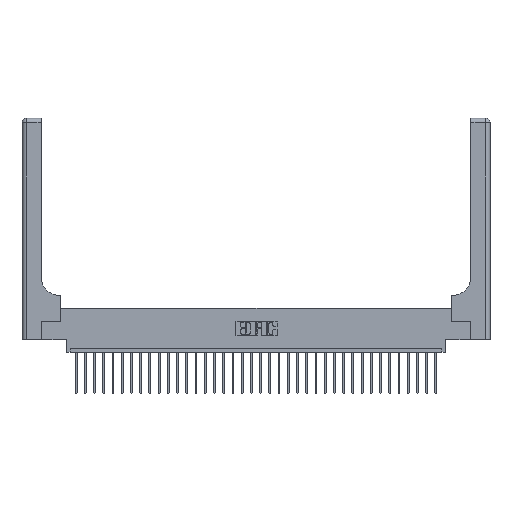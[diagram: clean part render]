
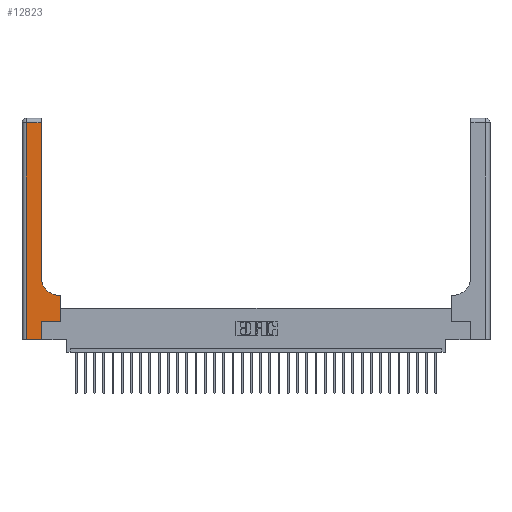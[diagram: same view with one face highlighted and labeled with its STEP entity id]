
A CAD part, top view. The second image highlights one B-rep face of the part: STEP entity #12823.
In plain terms, the highlighted planar face has unit normal (0, 0, 1).
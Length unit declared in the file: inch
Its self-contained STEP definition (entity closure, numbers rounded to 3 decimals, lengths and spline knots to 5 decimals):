
#86 = LINE ( 'NONE', #18781, #7908 ) ;
#174 = DIRECTION ( 'NONE',  ( -1., 0., 0. ) ) ;
#905 = PLANE ( 'NONE',  #30037 ) ;
#2286 = LINE ( 'NONE', #4970, #17020 ) ;
#3731 = DIRECTION ( 'NONE',  ( -1., 0., 0. ) ) ;
#4066 = CARTESIAN_POINT ( 'NONE',  ( 0.26, 2.94, 0.37 ) ) ;
#4112 = VERTEX_POINT ( 'NONE', #7474 ) ;
#4348 = LINE ( 'NONE', #20897, #28517 ) ;
#4426 = VERTEX_POINT ( 'NONE', #4066 ) ;
#4915 = CARTESIAN_POINT ( 'NONE',  ( 0.06, 2.94, 0.37 ) ) ;
#4970 = CARTESIAN_POINT ( 'NONE',  ( 0.528, 0.25, 0.37 ) ) ;
#6006 = DIRECTION ( 'NONE',  ( 0., 0., -1. ) ) ;
#6823 = VERTEX_POINT ( 'NONE', #7811 ) ;
#6849 = ORIENTED_EDGE ( 'NONE', *, *, #12622, .T. ) ;
#7474 = CARTESIAN_POINT ( 'NONE',  ( 0.265, 0., 0.37 ) ) ;
#7811 = CARTESIAN_POINT ( 'NONE',  ( 0.528, 0.25, 0.37 ) ) ;
#7908 = VECTOR ( 'NONE', #9663, 39.37008 ) ;
#8454 = EDGE_CURVE ( 'NONE', #21024, #4426, #19299, .T. ) ;
#9227 = CARTESIAN_POINT ( 'NONE',  ( 0.265, 0.25, 0.37 ) ) ;
#9582 = ORIENTED_EDGE ( 'NONE', *, *, #11792, .T. ) ;
#9663 = DIRECTION ( 'NONE',  ( 0., -1., 0. ) ) ;
#11144 = ORIENTED_EDGE ( 'NONE', *, *, #14262, .T. ) ;
#11792 = EDGE_CURVE ( 'NONE', #28270, #6823, #13527, .T. ) ;
#12622 = EDGE_CURVE ( 'NONE', #4112, #28270, #4348, .T. ) ;
#12823 = ADVANCED_FACE ( 'NONE', ( #29595 ), #905, .F. ) ;
#12825 = VERTEX_POINT ( 'NONE', #13071 ) ;
#12966 = VERTEX_POINT ( 'NONE', #19039 ) ;
#13030 = VECTOR ( 'NONE', #13961, 39.37008 ) ;
#13071 = CARTESIAN_POINT ( 'NONE',  ( 0.528, 0.6, 0.37 ) ) ;
#13268 = CIRCLE ( 'NONE', #25386, 0.25 ) ;
#13359 = VECTOR ( 'NONE', #27005, 39.37008 ) ;
#13527 = LINE ( 'NONE', #27594, #27817 ) ;
#13961 = DIRECTION ( 'NONE',  ( 0., 1., 0. ) ) ;
#14262 = EDGE_CURVE ( 'NONE', #4426, #24753, #20369, .T. ) ;
#14575 = EDGE_CURVE ( 'NONE', #6823, #12825, #2286, .T. ) ;
#15204 = ORIENTED_EDGE ( 'NONE', *, *, #19907, .T. ) ;
#15368 = CARTESIAN_POINT ( 'NONE',  ( 0., 2.94, 0.37 ) ) ;
#15503 = EDGE_CURVE ( 'NONE', #12966, #21024, #13268, .T. ) ;
#16274 = EDGE_CURVE ( 'NONE', #12825, #12966, #25276, .T. ) ;
#16343 = ORIENTED_EDGE ( 'NONE', *, *, #16274, .T. ) ;
#16352 = CARTESIAN_POINT ( 'NONE',  ( 0., 0., 0.37 ) ) ;
#16463 = ORIENTED_EDGE ( 'NONE', *, *, #14575, .T. ) ;
#17020 = VECTOR ( 'NONE', #26473, 39.37008 ) ;
#18781 = CARTESIAN_POINT ( 'NONE',  ( 0.06, 3., 0.37 ) ) ;
#19039 = CARTESIAN_POINT ( 'NONE',  ( 0.51, 0.6, 0.37 ) ) ;
#19051 = ORIENTED_EDGE ( 'NONE', *, *, #8454, .T. ) ;
#19299 = LINE ( 'NONE', #20740, #13030 ) ;
#19511 = EDGE_CURVE ( 'NONE', #24753, #30418, #86, .T. ) ;
#19907 = EDGE_CURVE ( 'NONE', #30418, #4112, #30331, .T. ) ;
#20080 = CARTESIAN_POINT ( 'NONE',  ( 0., 3., 0.37 ) ) ;
#20369 = LINE ( 'NONE', #15368, #13359 ) ;
#20678 = DIRECTION ( 'NONE',  ( 1., 0., 0. ) ) ;
#20740 = CARTESIAN_POINT ( 'NONE',  ( 0.26, 3., 0.37 ) ) ;
#20897 = CARTESIAN_POINT ( 'NONE',  ( 0.265, 0., 0.37 ) ) ;
#21024 = VERTEX_POINT ( 'NONE', #25613 ) ;
#21196 = CARTESIAN_POINT ( 'NONE',  ( 0.51, 0.85, 0.37 ) ) ;
#21583 = VECTOR ( 'NONE', #20678, 39.37008 ) ;
#22731 = VECTOR ( 'NONE', #174, 39.37008 ) ;
#22961 = EDGE_LOOP ( 'NONE', ( #19051, #11144, #27529, #15204, #6849, #9582, #16463, #16343, #30159 ) ) ;
#23328 = DIRECTION ( 'NONE',  ( 0., 1., 0. ) ) ;
#23730 = DIRECTION ( 'NONE',  ( 1., 0., 0. ) ) ;
#23828 = CARTESIAN_POINT ( 'NONE',  ( 0.26, 0.6, 0.37 ) ) ;
#24753 = VERTEX_POINT ( 'NONE', #4915 ) ;
#25276 = LINE ( 'NONE', #23828, #22731 ) ;
#25386 = AXIS2_PLACEMENT_3D ( 'NONE', #21196, #28212, #23730 ) ;
#25529 = DIRECTION ( 'NONE',  ( 1., 0., 0. ) ) ;
#25613 = CARTESIAN_POINT ( 'NONE',  ( 0.26, 0.85, 0.37 ) ) ;
#26473 = DIRECTION ( 'NONE',  ( 0., 1., 0. ) ) ;
#27005 = DIRECTION ( 'NONE',  ( -1., 0., 0. ) ) ;
#27529 = ORIENTED_EDGE ( 'NONE', *, *, #19511, .T. ) ;
#27594 = CARTESIAN_POINT ( 'NONE',  ( 0.265, 0.25, 0.37 ) ) ;
#27678 = CARTESIAN_POINT ( 'NONE',  ( 0.06, 0., 0.37 ) ) ;
#27817 = VECTOR ( 'NONE', #25529, 39.37008 ) ;
#28212 = DIRECTION ( 'NONE',  ( 0., 0., -1. ) ) ;
#28270 = VERTEX_POINT ( 'NONE', #9227 ) ;
#28517 = VECTOR ( 'NONE', #23328, 39.37008 ) ;
#29595 = FACE_OUTER_BOUND ( 'NONE', #22961, .T. ) ;
#30037 = AXIS2_PLACEMENT_3D ( 'NONE', #20080, #6006, #3731 ) ;
#30159 = ORIENTED_EDGE ( 'NONE', *, *, #15503, .T. ) ;
#30331 = LINE ( 'NONE', #16352, #21583 ) ;
#30418 = VERTEX_POINT ( 'NONE', #27678 ) ;
